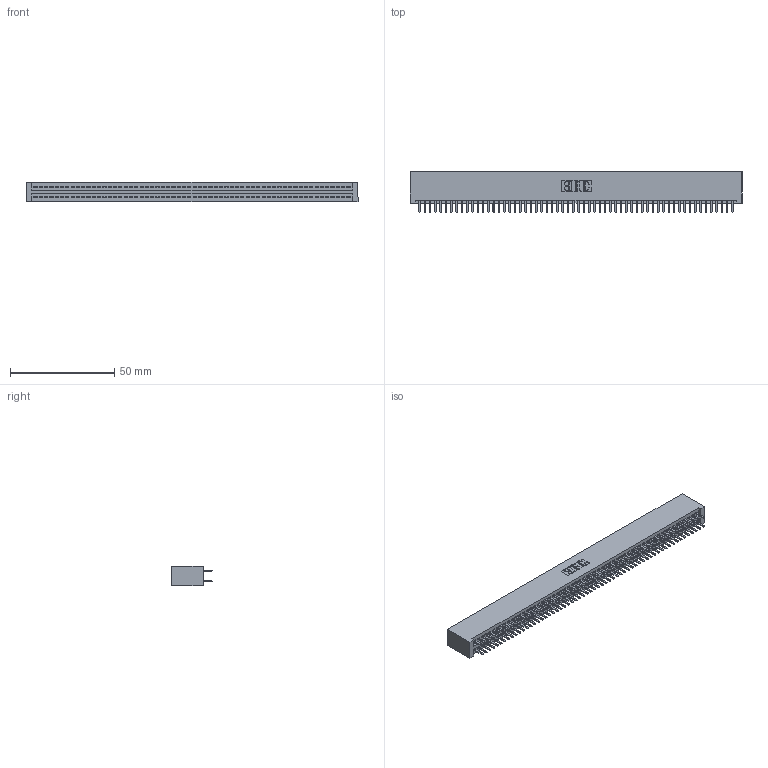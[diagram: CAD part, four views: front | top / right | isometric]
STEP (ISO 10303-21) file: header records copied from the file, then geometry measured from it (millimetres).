
FILE_DESCRIPTION (( 'STEP AP203' ), '1' );
FILE_NAME ('395-120-520-201.STEP', '2019-10-28T03:30:09', ( '' ), ( '' ), 'SwSTEP 2.0', 'SolidWorks 2016', '' );
FILE_SCHEMA (( 'CONFIG_CONTROL_DESIGN' ));
Length unit declared in the file: inch
Products named in the file (3): 345 Part_No Mounting Lugs; 345-292-001_345-293-120; 395-120-520-201
Assembly tree (121 placements, depth 2):
  395-120-520-201
    345 Part_No Mounting Lugs
    345-292-001_345-293-120  x120
Bounding box: 159 x 19.68 x 9.4 mm (x, y, z)
Volume: 16176 mm3; surface area: 24450.6 mm2
Topology: 121 solids, 121 shells, 6598 faces, 19157 edges, 12450 vertices
Faces by surface type: plane 4276, cylinder 2322
Entity records: 44491 total; most frequent: CARTESIAN_POINT 7452, ORIENTED_EDGE 7374, DIRECTION 6531, EDGE_CURVE 3687, VECTOR 3319, LINE 3319, VERTEX_POINT 2454, AXIS2_PLACEMENT_3D 1606
